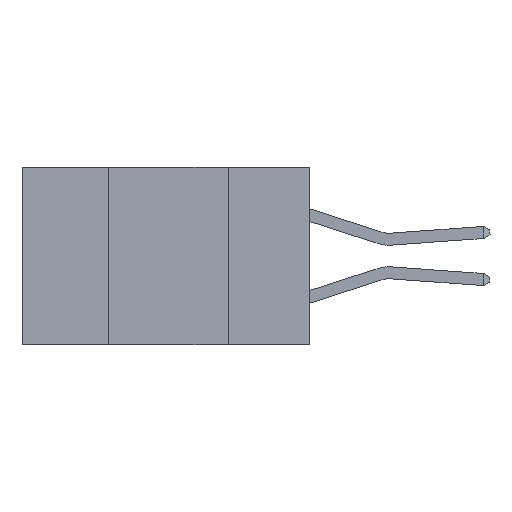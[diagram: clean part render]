
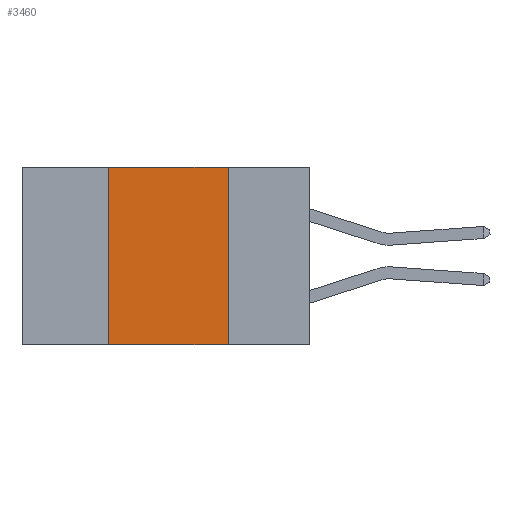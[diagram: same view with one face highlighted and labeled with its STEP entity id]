
A CAD part, left-side view. The second image highlights one B-rep face of the part: STEP entity #3460.
In plain terms, the highlighted planar face has unit normal (-1, 0, 0).
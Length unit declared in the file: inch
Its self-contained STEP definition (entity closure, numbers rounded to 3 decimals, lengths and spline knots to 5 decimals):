
#49 = CARTESIAN_POINT ( 'NONE',  ( 0., 0.42, 0. ) ) ;
#364 = CARTESIAN_POINT ( 'NONE',  ( 0., 0.17, -0.37 ) ) ;
#1545 = LINE ( 'NONE', #3613, #9671 ) ;
#1621 = DIRECTION ( 'NONE',  ( 1., 0., 0. ) ) ;
#1981 = CARTESIAN_POINT ( 'NONE',  ( 0., 0.6, 0. ) ) ;
#3091 = CARTESIAN_POINT ( 'NONE',  ( 0., 0.17, 0. ) ) ;
#3460 = ADVANCED_FACE ( 'NONE', ( #4907 ), #10160, .F. ) ;
#3613 = CARTESIAN_POINT ( 'NONE',  ( 0., 0.42, 0. ) ) ;
#4414 = VERTEX_POINT ( 'NONE', #3091 ) ;
#4687 = VERTEX_POINT ( 'NONE', #49 ) ;
#4907 = FACE_OUTER_BOUND ( 'NONE', #5801, .T. ) ;
#5307 = DIRECTION ( 'NONE',  ( 0., -1., 0. ) ) ;
#5447 = EDGE_CURVE ( 'NONE', #10869, #5738, #11382, .T. ) ;
#5702 = EDGE_CURVE ( 'NONE', #4414, #5738, #8530, .T. ) ;
#5738 = VERTEX_POINT ( 'NONE', #364 ) ;
#5801 = EDGE_LOOP ( 'NONE', ( #8838, #12425, #7997, #11660 ) ) ;
#5817 = VECTOR ( 'NONE', #12433, 39.37008 ) ;
#7997 = ORIENTED_EDGE ( 'NONE', *, *, #12144, .F. ) ;
#8530 = LINE ( 'NONE', #13100, #5817 ) ;
#8703 = VECTOR ( 'NONE', #10407, 39.37008 ) ;
#8838 = ORIENTED_EDGE ( 'NONE', *, *, #5702, .F. ) ;
#9342 = DIRECTION ( 'NONE',  ( 0., 0., -1. ) ) ;
#9435 = CARTESIAN_POINT ( 'NONE',  ( 0., 0.6, 0. ) ) ;
#9671 = VECTOR ( 'NONE', #12840, 39.37008 ) ;
#9990 = CARTESIAN_POINT ( 'NONE',  ( 0., 0.6, -0.37 ) ) ;
#10028 = VECTOR ( 'NONE', #5307, 39.37008 ) ;
#10160 = PLANE ( 'NONE',  #12787 ) ;
#10407 = DIRECTION ( 'NONE',  ( 0., -1., 0. ) ) ;
#10834 = EDGE_CURVE ( 'NONE', #4687, #4414, #12928, .T. ) ;
#10869 = VERTEX_POINT ( 'NONE', #11439 ) ;
#11382 = LINE ( 'NONE', #9990, #8703 ) ;
#11439 = CARTESIAN_POINT ( 'NONE',  ( 0., 0.42, -0.37 ) ) ;
#11660 = ORIENTED_EDGE ( 'NONE', *, *, #5447, .T. ) ;
#12144 = EDGE_CURVE ( 'NONE', #10869, #4687, #1545, .T. ) ;
#12425 = ORIENTED_EDGE ( 'NONE', *, *, #10834, .F. ) ;
#12433 = DIRECTION ( 'NONE',  ( 0., 0., -1. ) ) ;
#12787 = AXIS2_PLACEMENT_3D ( 'NONE', #1981, #1621, #9342 ) ;
#12840 = DIRECTION ( 'NONE',  ( 0., 0., 1. ) ) ;
#12928 = LINE ( 'NONE', #9435, #10028 ) ;
#13100 = CARTESIAN_POINT ( 'NONE',  ( 0., 0.17, 0. ) ) ;
